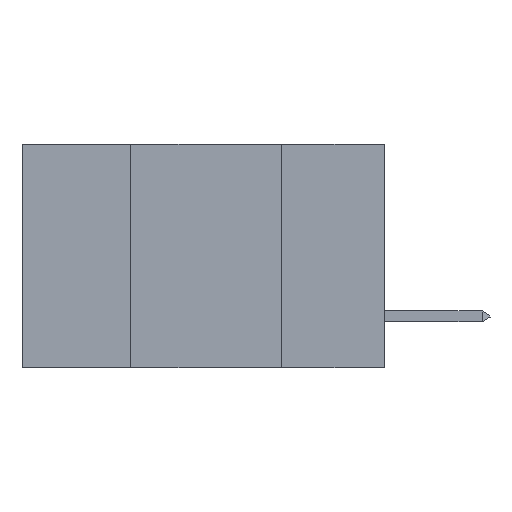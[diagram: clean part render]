
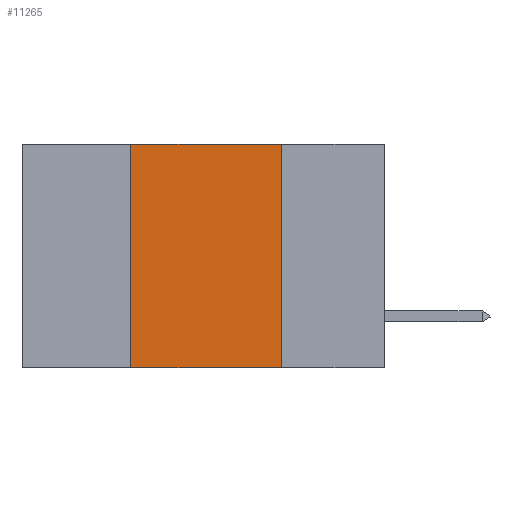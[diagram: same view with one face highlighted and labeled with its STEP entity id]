
A CAD part, left-side view. The second image highlights one B-rep face of the part: STEP entity #11265.
In plain terms, the highlighted planar face has unit normal (-1, 0, 0).
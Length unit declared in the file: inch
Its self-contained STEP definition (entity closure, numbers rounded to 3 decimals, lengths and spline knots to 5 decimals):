
#42 = CARTESIAN_POINT ( 'NONE',  ( 0., 0.17, -0.37 ) ) ;
#43 = DIRECTION ( 'NONE',  ( 0., 0., -1. ) ) ;
#841 = VECTOR ( 'NONE', #43, 39.37008 ) ;
#1422 = LINE ( 'NONE', #3679, #841 ) ;
#1473 = CARTESIAN_POINT ( 'NONE',  ( 0., 0.42, 0. ) ) ;
#1527 = CARTESIAN_POINT ( 'NONE',  ( 0., 0.42, -0.37 ) ) ;
#2265 = CARTESIAN_POINT ( 'NONE',  ( 0., 0.6, -0.37 ) ) ;
#3056 = VECTOR ( 'NONE', #13151, 39.37008 ) ;
#3171 = VERTEX_POINT ( 'NONE', #42 ) ;
#3679 = CARTESIAN_POINT ( 'NONE',  ( 0., 0.17, 0. ) ) ;
#4767 = EDGE_CURVE ( 'NONE', #5657, #12819, #8413, .T. ) ;
#4902 = CARTESIAN_POINT ( 'NONE',  ( 0., 0.6, 0. ) ) ;
#4965 = DIRECTION ( 'NONE',  ( 0., 0., -1. ) ) ;
#5294 = ORIENTED_EDGE ( 'NONE', *, *, #8341, .F. ) ;
#5657 = VERTEX_POINT ( 'NONE', #1473 ) ;
#5915 = EDGE_LOOP ( 'NONE', ( #5294, #6101, #15150, #14895 ) ) ;
#5938 = DIRECTION ( 'NONE',  ( 0., 0., 1. ) ) ;
#6091 = DIRECTION ( 'NONE',  ( 1., 0., 0. ) ) ;
#6101 = ORIENTED_EDGE ( 'NONE', *, *, #4767, .F. ) ;
#7336 = CARTESIAN_POINT ( 'NONE',  ( 0., 0.17, 0. ) ) ;
#8341 = EDGE_CURVE ( 'NONE', #12819, #3171, #1422, .T. ) ;
#8413 = LINE ( 'NONE', #9443, #3056 ) ;
#9318 = EDGE_CURVE ( 'NONE', #15661, #5657, #15509, .T. ) ;
#9443 = CARTESIAN_POINT ( 'NONE',  ( 0., 0.6, 0. ) ) ;
#9865 = EDGE_CURVE ( 'NONE', #15661, #3171, #15598, .T. ) ;
#10749 = VECTOR ( 'NONE', #5938, 39.37008 ) ;
#11242 = VECTOR ( 'NONE', #14517, 39.37008 ) ;
#11265 = ADVANCED_FACE ( 'NONE', ( #15272 ), #13576, .F. ) ;
#12103 = CARTESIAN_POINT ( 'NONE',  ( 0., 0.42, 0. ) ) ;
#12819 = VERTEX_POINT ( 'NONE', #7336 ) ;
#13151 = DIRECTION ( 'NONE',  ( 0., -1., 0. ) ) ;
#13576 = PLANE ( 'NONE',  #14418 ) ;
#14418 = AXIS2_PLACEMENT_3D ( 'NONE', #4902, #6091, #4965 ) ;
#14517 = DIRECTION ( 'NONE',  ( 0., -1., 0. ) ) ;
#14895 = ORIENTED_EDGE ( 'NONE', *, *, #9865, .T. ) ;
#15150 = ORIENTED_EDGE ( 'NONE', *, *, #9318, .F. ) ;
#15272 = FACE_OUTER_BOUND ( 'NONE', #5915, .T. ) ;
#15509 = LINE ( 'NONE', #12103, #10749 ) ;
#15598 = LINE ( 'NONE', #2265, #11242 ) ;
#15661 = VERTEX_POINT ( 'NONE', #1527 ) ;
